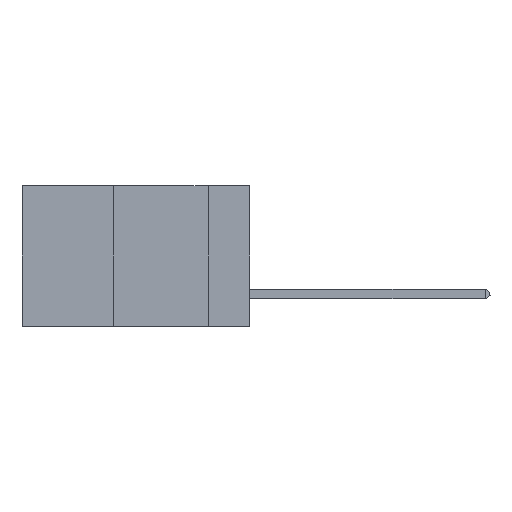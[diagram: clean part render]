
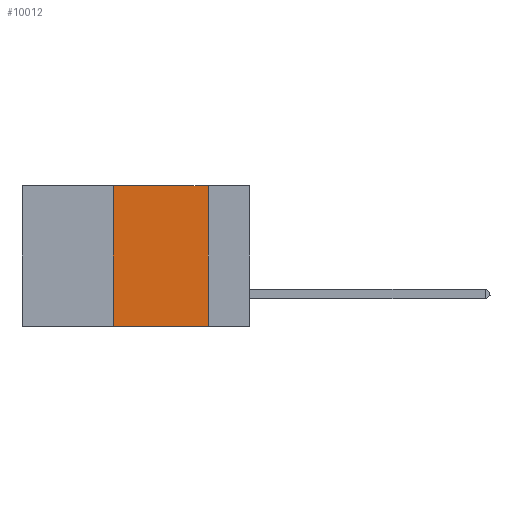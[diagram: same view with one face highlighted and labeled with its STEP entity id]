
A CAD part, left-side view. The second image highlights one B-rep face of the part: STEP entity #10012.
In plain terms, the highlighted planar face has unit normal (-1, 0, 0).
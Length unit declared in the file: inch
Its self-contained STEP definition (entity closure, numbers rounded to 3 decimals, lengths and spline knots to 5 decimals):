
#385 = DIRECTION ( 'NONE',  ( 0., 0., 1. ) ) ;
#1158 = ORIENTED_EDGE ( 'NONE', *, *, #19782, .F. ) ;
#1703 = VECTOR ( 'NONE', #19035, 39.37008 ) ;
#1848 = ORIENTED_EDGE ( 'NONE', *, *, #17319, .T. ) ;
#2202 = CARTESIAN_POINT ( 'NONE',  ( 0., 0.36, 0. ) ) ;
#2216 = CARTESIAN_POINT ( 'NONE',  ( 0., 0.36, 0. ) ) ;
#2456 = CARTESIAN_POINT ( 'NONE',  ( 0., 0.11, 0. ) ) ;
#3500 = AXIS2_PLACEMENT_3D ( 'NONE', #17010, #6622, #18780 ) ;
#4140 = VECTOR ( 'NONE', #14425, 39.37008 ) ;
#4883 = PLANE ( 'NONE',  #3500 ) ;
#6622 = DIRECTION ( 'NONE',  ( 1., 0., 0. ) ) ;
#7423 = VERTEX_POINT ( 'NONE', #16645 ) ;
#8067 = EDGE_CURVE ( 'NONE', #14088, #20050, #17166, .T. ) ;
#10012 = ADVANCED_FACE ( 'NONE', ( #20916 ), #4883, .F. ) ;
#10628 = LINE ( 'NONE', #2202, #17431 ) ;
#10646 = CARTESIAN_POINT ( 'NONE',  ( 0., 0.6, -0.37 ) ) ;
#11280 = EDGE_LOOP ( 'NONE', ( #18620, #17331, #1158, #1848 ) ) ;
#13100 = VERTEX_POINT ( 'NONE', #17907 ) ;
#13365 = LINE ( 'NONE', #2456, #4140 ) ;
#14088 = VERTEX_POINT ( 'NONE', #2216 ) ;
#14143 = DIRECTION ( 'NONE',  ( 0., -1., 0. ) ) ;
#14425 = DIRECTION ( 'NONE',  ( 0., 0., -1. ) ) ;
#15994 = EDGE_CURVE ( 'NONE', #20050, #7423, #13365, .T. ) ;
#16645 = CARTESIAN_POINT ( 'NONE',  ( 0., 0.11, -0.37 ) ) ;
#16852 = LINE ( 'NONE', #10646, #18212 ) ;
#17010 = CARTESIAN_POINT ( 'NONE',  ( 0., 0.6, 0. ) ) ;
#17166 = LINE ( 'NONE', #22218, #1703 ) ;
#17319 = EDGE_CURVE ( 'NONE', #13100, #7423, #16852, .T. ) ;
#17331 = ORIENTED_EDGE ( 'NONE', *, *, #8067, .F. ) ;
#17431 = VECTOR ( 'NONE', #385, 39.37008 ) ;
#17907 = CARTESIAN_POINT ( 'NONE',  ( 0., 0.36, -0.37 ) ) ;
#18040 = CARTESIAN_POINT ( 'NONE',  ( 0., 0.11, 0. ) ) ;
#18212 = VECTOR ( 'NONE', #14143, 39.37008 ) ;
#18620 = ORIENTED_EDGE ( 'NONE', *, *, #15994, .F. ) ;
#18780 = DIRECTION ( 'NONE',  ( 0., 0., -1. ) ) ;
#19035 = DIRECTION ( 'NONE',  ( 0., -1., 0. ) ) ;
#19782 = EDGE_CURVE ( 'NONE', #13100, #14088, #10628, .T. ) ;
#20050 = VERTEX_POINT ( 'NONE', #18040 ) ;
#20916 = FACE_OUTER_BOUND ( 'NONE', #11280, .T. ) ;
#22218 = CARTESIAN_POINT ( 'NONE',  ( 0., 0.6, 0. ) ) ;
